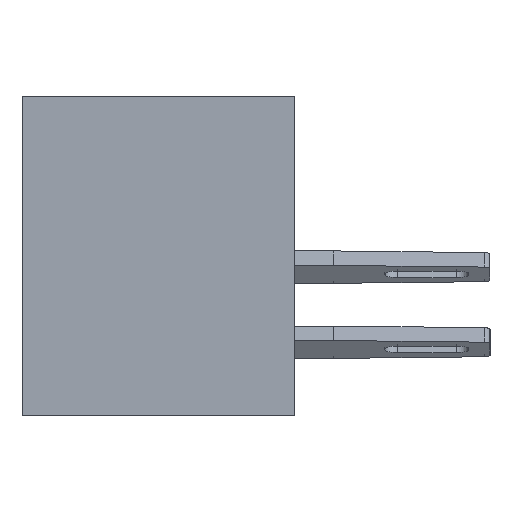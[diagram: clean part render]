
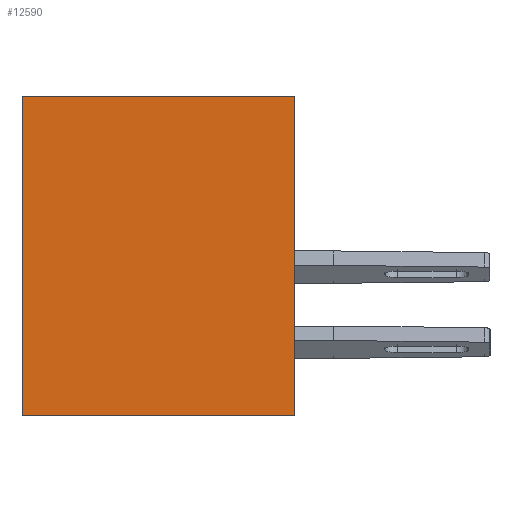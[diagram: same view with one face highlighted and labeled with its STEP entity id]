
A CAD part, left-side view. The second image highlights one B-rep face of the part: STEP entity #12590.
In plain terms, the highlighted planar face has unit normal (-1, 0, 0).
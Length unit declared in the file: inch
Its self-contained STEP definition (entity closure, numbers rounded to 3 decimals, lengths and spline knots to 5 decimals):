
#198 = CARTESIAN_POINT ( 'NONE',  ( 0., 0., -0.531 ) ) ;
#263 = EDGE_CURVE ( 'NONE', #21143, #14669, #22384, .T. ) ;
#908 = VECTOR ( 'NONE', #18033, 39.37008 ) ;
#942 = CARTESIAN_POINT ( 'NONE',  ( 0., 0.453, 0. ) ) ;
#1234 = VECTOR ( 'NONE', #2624, 39.37008 ) ;
#1684 = VERTEX_POINT ( 'NONE', #198 ) ;
#1712 = FACE_OUTER_BOUND ( 'NONE', #16175, .T. ) ;
#2624 = DIRECTION ( 'NONE',  ( 0., -1., 0. ) ) ;
#3125 = CARTESIAN_POINT ( 'NONE',  ( 0., 0.453, 0. ) ) ;
#3309 = ORIENTED_EDGE ( 'NONE', *, *, #263, .F. ) ;
#4412 = VECTOR ( 'NONE', #10948, 39.37008 ) ;
#5819 = AXIS2_PLACEMENT_3D ( 'NONE', #7627, #7451, #15772 ) ;
#7451 = DIRECTION ( 'NONE',  ( 1., 0., 0. ) ) ;
#7481 = VERTEX_POINT ( 'NONE', #11349 ) ;
#7627 = CARTESIAN_POINT ( 'NONE',  ( 0., 0.453, 0. ) ) ;
#9678 = PLANE ( 'NONE',  #5819 ) ;
#9889 = LINE ( 'NONE', #19858, #908 ) ;
#10948 = DIRECTION ( 'NONE',  ( 0., -1., 0. ) ) ;
#11015 = ORIENTED_EDGE ( 'NONE', *, *, #15049, .T. ) ;
#11349 = CARTESIAN_POINT ( 'NONE',  ( 0., 0.453, -0.531 ) ) ;
#12397 = ORIENTED_EDGE ( 'NONE', *, *, #13615, .F. ) ;
#12590 = ADVANCED_FACE ( 'NONE', ( #1712 ), #9678, .F. ) ;
#12800 = LINE ( 'NONE', #17050, #1234 ) ;
#13615 = EDGE_CURVE ( 'NONE', #7481, #21143, #18949, .T. ) ;
#14669 = VERTEX_POINT ( 'NONE', #17258 ) ;
#14845 = DIRECTION ( 'NONE',  ( 0., 0., 1. ) ) ;
#15049 = EDGE_CURVE ( 'NONE', #7481, #1684, #12800, .T. ) ;
#15772 = DIRECTION ( 'NONE',  ( 0., 0., -1. ) ) ;
#16175 = EDGE_LOOP ( 'NONE', ( #24448, #3309, #12397, #11015 ) ) ;
#17050 = CARTESIAN_POINT ( 'NONE',  ( 0., 0.453, -0.531 ) ) ;
#17258 = CARTESIAN_POINT ( 'NONE',  ( 0., 0., 0. ) ) ;
#18033 = DIRECTION ( 'NONE',  ( 0., 0., 1. ) ) ;
#18949 = LINE ( 'NONE', #23448, #23150 ) ;
#19858 = CARTESIAN_POINT ( 'NONE',  ( 0., 0., 0. ) ) ;
#21143 = VERTEX_POINT ( 'NONE', #942 ) ;
#22384 = LINE ( 'NONE', #3125, #4412 ) ;
#23150 = VECTOR ( 'NONE', #14845, 39.37008 ) ;
#23448 = CARTESIAN_POINT ( 'NONE',  ( 0., 0.453, 0. ) ) ;
#24448 = ORIENTED_EDGE ( 'NONE', *, *, #24546, .T. ) ;
#24546 = EDGE_CURVE ( 'NONE', #1684, #14669, #9889, .T. ) ;
